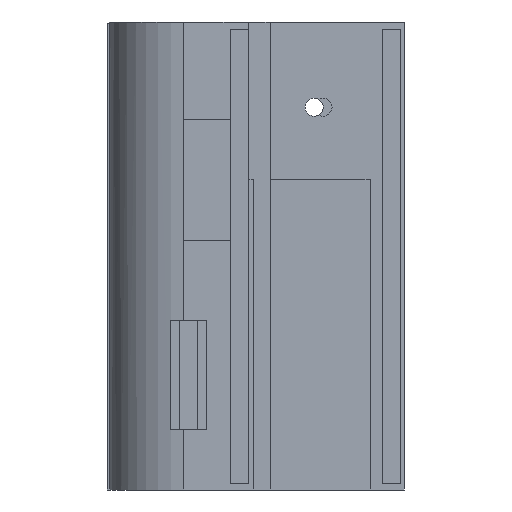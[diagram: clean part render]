
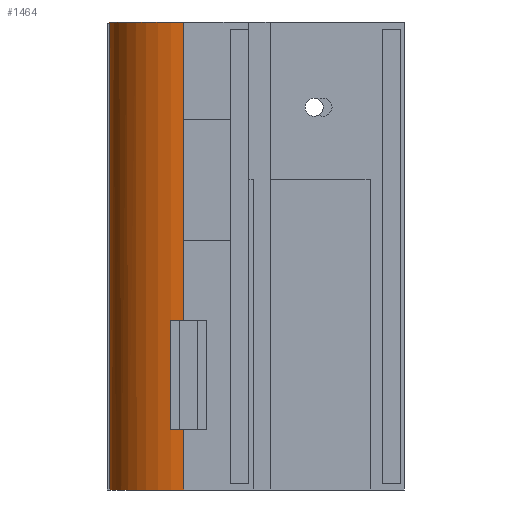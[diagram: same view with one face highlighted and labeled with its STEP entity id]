
A CAD part, left-side view. The second image highlights one B-rep face of the part: STEP entity #1464.
In plain terms, the highlighted cylindrical face has radius 13 mm (diameter 26 mm), a partial arc.
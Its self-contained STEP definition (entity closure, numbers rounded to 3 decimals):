
#206 = CARTESIAN_POINT ( 'NONE',  ( -1.5, 37.913, -1. ) ) ;
#312 = EDGE_CURVE ( 'NONE', #2949, #5010, #5995, .T. ) ;
#599 = ORIENTED_EDGE ( 'NONE', *, *, #1990, .T. ) ;
#612 = DIRECTION ( 'NONE',  ( 0., 0., -1. ) ) ;
#615 = DIRECTION ( 'NONE',  ( 1., 0., 0. ) ) ;
#640 = DIRECTION ( 'NONE',  ( 0., 0., -1. ) ) ;
#786 = CIRCLE ( 'NONE', #3017, 13. ) ;
#978 = DIRECTION ( 'NONE',  ( 0., 0., -1. ) ) ;
#986 = ORIENTED_EDGE ( 'NONE', *, *, #6208, .F. ) ;
#1130 = EDGE_CURVE ( 'NONE', #4664, #7276, #5014, .T. ) ;
#1271 = CARTESIAN_POINT ( 'NONE',  ( 0., 25., -1. ) ) ;
#1346 = VECTOR ( 'NONE', #612, 1000. ) ;
#1464 = ADVANCED_FACE ( 'NONE', ( #4512 ), #3161, .T. ) ;
#1733 = AXIS2_PLACEMENT_3D ( 'NONE', #1271, #7120, #615 ) ;
#1783 = CARTESIAN_POINT ( 'NONE',  ( 11., 31.928, -1. ) ) ;
#1807 = CARTESIAN_POINT ( 'NONE',  ( -11., 31.928, -1. ) ) ;
#1841 = CARTESIAN_POINT ( 'NONE',  ( 0., 25., -1. ) ) ;
#1990 = EDGE_CURVE ( 'NONE', #2949, #7690, #5186, .T. ) ;
#1992 = ORIENTED_EDGE ( 'NONE', *, *, #3720, .F. ) ;
#2055 = VECTOR ( 'NONE', #2349, 1000. ) ;
#2175 = VERTEX_POINT ( 'NONE', #206 ) ;
#2187 = CARTESIAN_POINT ( 'NONE',  ( -12.982, 25.692, -1. ) ) ;
#2223 = CARTESIAN_POINT ( 'NONE',  ( -1.5, 37.913, -1. ) ) ;
#2285 = DIRECTION ( 'NONE',  ( 1., 0., 0. ) ) ;
#2349 = DIRECTION ( 'NONE',  ( 0., 0., 1. ) ) ;
#2354 = DIRECTION ( 'NONE',  ( 0., 0., -1. ) ) ;
#2360 = EDGE_CURVE ( 'NONE', #7690, #7276, #2626, .T. ) ;
#2393 = CARTESIAN_POINT ( 'NONE',  ( -12.982, 25.692, -1. ) ) ;
#2626 = CIRCLE ( 'NONE', #6392, 13. ) ;
#2664 = CARTESIAN_POINT ( 'NONE',  ( 1.5, 37.913, -1. ) ) ;
#2818 = VERTEX_POINT ( 'NONE', #6070 ) ;
#2949 = VERTEX_POINT ( 'NONE', #2187 ) ;
#3017 = AXIS2_PLACEMENT_3D ( 'NONE', #3144, #7800, #4498 ) ;
#3077 = AXIS2_PLACEMENT_3D ( 'NONE', #4863, #978, #2285 ) ;
#3144 = CARTESIAN_POINT ( 'NONE',  ( 0., 25., -1. ) ) ;
#3161 = CYLINDRICAL_SURFACE ( 'NONE', #8451, 13. ) ;
#3250 = CARTESIAN_POINT ( 'NONE',  ( 0., 25., -1. ) ) ;
#3450 = VERTEX_POINT ( 'NONE', #5826 ) ;
#3614 = VECTOR ( 'NONE', #2354, 1000. ) ;
#3707 = AXIS2_PLACEMENT_3D ( 'NONE', #1841, #4508, #7166 ) ;
#3720 = EDGE_CURVE ( 'NONE', #2818, #7316, #5158, .T. ) ;
#3781 = DIRECTION ( 'NONE',  ( 0., 0., -1. ) ) ;
#4003 = CARTESIAN_POINT ( 'NONE',  ( 0., 25., 76.189 ) ) ;
#4325 = CARTESIAN_POINT ( 'NONE',  ( -12.982, 25.692, 76.189 ) ) ;
#4328 = CARTESIAN_POINT ( 'NONE',  ( 12.986, 25.605, -1. ) ) ;
#4498 = DIRECTION ( 'NONE',  ( 1., 0., 0. ) ) ;
#4508 = DIRECTION ( 'NONE',  ( 0., 0., -1. ) ) ;
#4512 = FACE_OUTER_BOUND ( 'NONE', #5110, .T. ) ;
#4664 = VERTEX_POINT ( 'NONE', #4328 ) ;
#4698 = EDGE_CURVE ( 'NONE', #7316, #3450, #6498, .T. ) ;
#4767 = EDGE_CURVE ( 'NONE', #5010, #2175, #786, .T. ) ;
#4863 = CARTESIAN_POINT ( 'NONE',  ( 0., 25., 76. ) ) ;
#5010 = VERTEX_POINT ( 'NONE', #1807 ) ;
#5014 = LINE ( 'NONE', #8491, #5526 ) ;
#5110 = EDGE_LOOP ( 'NONE', ( #5615, #599, #8403, #6730, #986, #7756, #7078, #1992, #7177, #7172 ) ) ;
#5112 = DIRECTION ( 'NONE',  ( 0., 0., -1. ) ) ;
#5143 = DIRECTION ( 'NONE',  ( 0., 0., 1. ) ) ;
#5158 = CIRCLE ( 'NONE', #3077, 13. ) ;
#5186 = LINE ( 'NONE', #2393, #2055 ) ;
#5526 = VECTOR ( 'NONE', #5143, 1000. ) ;
#5615 = ORIENTED_EDGE ( 'NONE', *, *, #312, .F. ) ;
#5826 = CARTESIAN_POINT ( 'NONE',  ( 1.5, 37.913, -1. ) ) ;
#5845 = EDGE_CURVE ( 'NONE', #3450, #7713, #8145, .T. ) ;
#5995 = CIRCLE ( 'NONE', #7113, 13. ) ;
#6041 = DIRECTION ( 'NONE',  ( 1., 0., 0. ) ) ;
#6070 = CARTESIAN_POINT ( 'NONE',  ( -1.5, 37.913, 76. ) ) ;
#6208 = EDGE_CURVE ( 'NONE', #7713, #4664, #8132, .T. ) ;
#6368 = LINE ( 'NONE', #2223, #3614 ) ;
#6392 = AXIS2_PLACEMENT_3D ( 'NONE', #4003, #640, #6041 ) ;
#6498 = LINE ( 'NONE', #2664, #1346 ) ;
#6555 = CARTESIAN_POINT ( 'NONE',  ( 0., 25., -1. ) ) ;
#6730 = ORIENTED_EDGE ( 'NONE', *, *, #1130, .F. ) ;
#6902 = CARTESIAN_POINT ( 'NONE',  ( 1.5, 37.913, 76. ) ) ;
#7075 = CARTESIAN_POINT ( 'NONE',  ( 12.986, 25.605, 76.189 ) ) ;
#7078 = ORIENTED_EDGE ( 'NONE', *, *, #4698, .F. ) ;
#7113 = AXIS2_PLACEMENT_3D ( 'NONE', #6555, #5112, #8547 ) ;
#7120 = DIRECTION ( 'NONE',  ( 0., 0., -1. ) ) ;
#7166 = DIRECTION ( 'NONE',  ( 1., 0., 0. ) ) ;
#7172 = ORIENTED_EDGE ( 'NONE', *, *, #4767, .F. ) ;
#7177 = ORIENTED_EDGE ( 'NONE', *, *, #7589, .T. ) ;
#7276 = VERTEX_POINT ( 'NONE', #7075 ) ;
#7316 = VERTEX_POINT ( 'NONE', #6902 ) ;
#7589 = EDGE_CURVE ( 'NONE', #2818, #2175, #6368, .T. ) ;
#7690 = VERTEX_POINT ( 'NONE', #4325 ) ;
#7713 = VERTEX_POINT ( 'NONE', #1783 ) ;
#7756 = ORIENTED_EDGE ( 'NONE', *, *, #5845, .F. ) ;
#7800 = DIRECTION ( 'NONE',  ( 0., 0., -1. ) ) ;
#7856 = DIRECTION ( 'NONE',  ( 1., 0., 0. ) ) ;
#8132 = CIRCLE ( 'NONE', #1733, 13. ) ;
#8145 = CIRCLE ( 'NONE', #3707, 13. ) ;
#8403 = ORIENTED_EDGE ( 'NONE', *, *, #2360, .T. ) ;
#8451 = AXIS2_PLACEMENT_3D ( 'NONE', #3250, #3781, #7856 ) ;
#8491 = CARTESIAN_POINT ( 'NONE',  ( 12.986, 25.605, -1. ) ) ;
#8547 = DIRECTION ( 'NONE',  ( 1., 0., 0. ) ) ;
